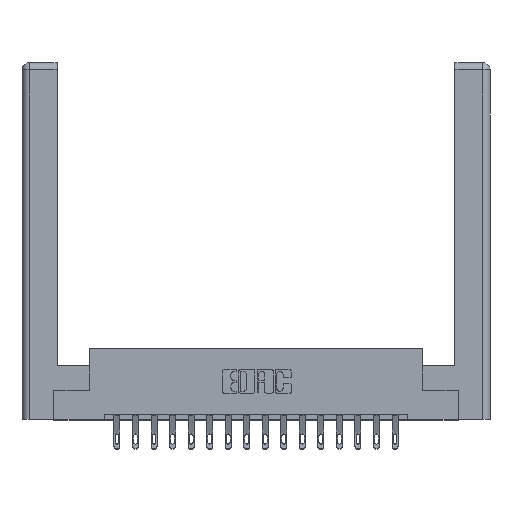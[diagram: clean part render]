
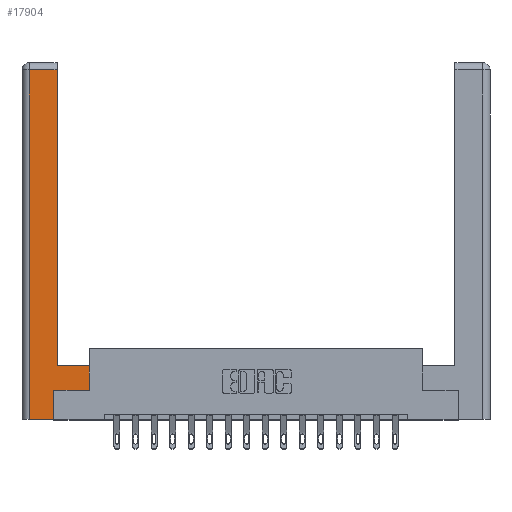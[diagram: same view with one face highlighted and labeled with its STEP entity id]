
A CAD part, top view. The second image highlights one B-rep face of the part: STEP entity #17904.
In plain terms, the highlighted planar face has unit normal (0, 0, 1).
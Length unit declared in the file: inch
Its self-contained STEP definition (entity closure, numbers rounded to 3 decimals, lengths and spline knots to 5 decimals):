
#75 = LINE ( 'NONE', #2359, #7084 ) ;
#76 = VERTEX_POINT ( 'NONE', #2235 ) ;
#370 = VERTEX_POINT ( 'NONE', #12340 ) ;
#673 = LINE ( 'NONE', #2169, #2218 ) ;
#685 = EDGE_CURVE ( 'NONE', #17061, #370, #15050, .T. ) ;
#923 = CARTESIAN_POINT ( 'NONE',  ( 0.565, 0.245, 0. ) ) ;
#997 = PLANE ( 'NONE',  #16231 ) ;
#1225 = VECTOR ( 'NONE', #3364, 39.37008 ) ;
#1628 = ORIENTED_EDGE ( 'NONE', *, *, #12150, .T. ) ;
#1632 = EDGE_CURVE ( 'NONE', #9701, #8899, #8459, .T. ) ;
#1858 = EDGE_CURVE ( 'NONE', #5154, #9964, #14301, .T. ) ;
#2169 = CARTESIAN_POINT ( 'NONE',  ( 0.565, 0.45, 0. ) ) ;
#2218 = VECTOR ( 'NONE', #10858, 39.37008 ) ;
#2235 = CARTESIAN_POINT ( 'NONE',  ( 0.565, 0.245, 0. ) ) ;
#2359 = CARTESIAN_POINT ( 'NONE',  ( 0.0615, 2.94, 0. ) ) ;
#2405 = VECTOR ( 'NONE', #6009, 39.37008 ) ;
#2899 = ORIENTED_EDGE ( 'NONE', *, *, #1858, .T. ) ;
#3364 = DIRECTION ( 'NONE',  ( 0., 1., 0. ) ) ;
#3552 = CARTESIAN_POINT ( 'NONE',  ( 0.0615, 0., 0. ) ) ;
#3696 = ORIENTED_EDGE ( 'NONE', *, *, #685, .T. ) ;
#3736 = EDGE_LOOP ( 'NONE', ( #7962, #5522, #2899, #1628, #13218, #8027, #9916, #3696 ) ) ;
#4928 = LINE ( 'NONE', #923, #9467 ) ;
#5154 = VERTEX_POINT ( 'NONE', #13821 ) ;
#5192 = EDGE_CURVE ( 'NONE', #370, #13682, #18284, .T. ) ;
#5195 = CARTESIAN_POINT ( 'NONE',  ( 0., 0., 0. ) ) ;
#5232 = CARTESIAN_POINT ( 'NONE',  ( 0.265, 0., 0. ) ) ;
#5522 = ORIENTED_EDGE ( 'NONE', *, *, #7547, .T. ) ;
#5557 = LINE ( 'NONE', #5232, #6713 ) ;
#6009 = DIRECTION ( 'NONE',  ( 0., 1., 0. ) ) ;
#6247 = CARTESIAN_POINT ( 'NONE',  ( 0.265, 0.245, 0. ) ) ;
#6451 = VECTOR ( 'NONE', #14181, 39.37008 ) ;
#6713 = VECTOR ( 'NONE', #6760, 39.37008 ) ;
#6729 = DIRECTION ( 'NONE',  ( 0., 0., -1. ) ) ;
#6760 = DIRECTION ( 'NONE',  ( 1., 0., 0. ) ) ;
#7084 = VECTOR ( 'NONE', #17249, 39.37008 ) ;
#7542 = CARTESIAN_POINT ( 'NONE',  ( 0.295, 3., 0. ) ) ;
#7547 = EDGE_CURVE ( 'NONE', #13682, #5154, #75, .T. ) ;
#7700 = CARTESIAN_POINT ( 'NONE',  ( 0.265, 0.245, 0. ) ) ;
#7962 = ORIENTED_EDGE ( 'NONE', *, *, #5192, .T. ) ;
#8027 = ORIENTED_EDGE ( 'NONE', *, *, #17038, .T. ) ;
#8459 = LINE ( 'NONE', #6247, #1225 ) ;
#8899 = VERTEX_POINT ( 'NONE', #7700 ) ;
#9156 = CARTESIAN_POINT ( 'NONE',  ( 0.0615, 0., 0. ) ) ;
#9457 = DIRECTION ( 'NONE',  ( 0., -1., 0. ) ) ;
#9467 = VECTOR ( 'NONE', #15458, 39.37008 ) ;
#9701 = VERTEX_POINT ( 'NONE', #15802 ) ;
#9916 = ORIENTED_EDGE ( 'NONE', *, *, #16919, .T. ) ;
#9964 = VERTEX_POINT ( 'NONE', #9156 ) ;
#10491 = VECTOR ( 'NONE', #9457, 39.37008 ) ;
#10858 = DIRECTION ( 'NONE',  ( 0., 1., 0. ) ) ;
#12150 = EDGE_CURVE ( 'NONE', #9964, #9701, #5557, .T. ) ;
#12340 = CARTESIAN_POINT ( 'NONE',  ( 0.295, 0.45, 0. ) ) ;
#12628 = DIRECTION ( 'NONE',  ( -1., 0., 0. ) ) ;
#13218 = ORIENTED_EDGE ( 'NONE', *, *, #1632, .T. ) ;
#13682 = VERTEX_POINT ( 'NONE', #16736 ) ;
#13821 = CARTESIAN_POINT ( 'NONE',  ( 0.0615, 2.94, 0. ) ) ;
#14181 = DIRECTION ( 'NONE',  ( -1., 0., 0. ) ) ;
#14301 = LINE ( 'NONE', #3552, #10491 ) ;
#15050 = LINE ( 'NONE', #17197, #6451 ) ;
#15458 = DIRECTION ( 'NONE',  ( 1., 0., 0. ) ) ;
#15802 = CARTESIAN_POINT ( 'NONE',  ( 0.265, 0., 0. ) ) ;
#16231 = AXIS2_PLACEMENT_3D ( 'NONE', #5195, #6729, #12628 ) ;
#16736 = CARTESIAN_POINT ( 'NONE',  ( 0.295, 2.94, 0. ) ) ;
#16919 = EDGE_CURVE ( 'NONE', #76, #17061, #673, .T. ) ;
#17038 = EDGE_CURVE ( 'NONE', #8899, #76, #4928, .T. ) ;
#17061 = VERTEX_POINT ( 'NONE', #18146 ) ;
#17197 = CARTESIAN_POINT ( 'NONE',  ( 0.295, 0.45, 0. ) ) ;
#17249 = DIRECTION ( 'NONE',  ( -1., 0., 0. ) ) ;
#17904 = ADVANCED_FACE ( 'NONE', ( #17951 ), #997, .F. ) ;
#17951 = FACE_OUTER_BOUND ( 'NONE', #3736, .T. ) ;
#18146 = CARTESIAN_POINT ( 'NONE',  ( 0.565, 0.45, 0. ) ) ;
#18284 = LINE ( 'NONE', #7542, #2405 ) ;
